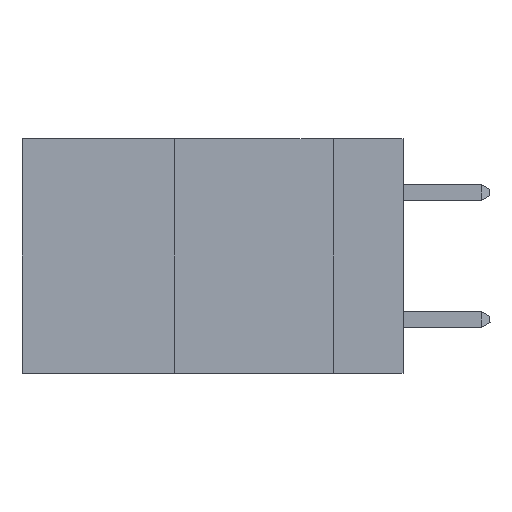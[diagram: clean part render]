
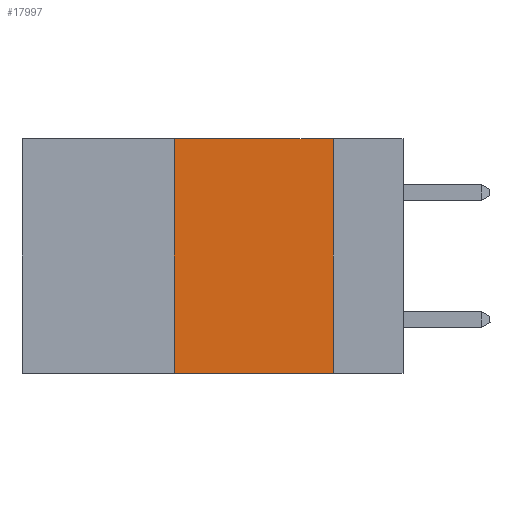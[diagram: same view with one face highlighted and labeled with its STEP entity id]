
A CAD part, left-side view. The second image highlights one B-rep face of the part: STEP entity #17997.
In plain terms, the highlighted planar face has unit normal (-1, 0, 0).
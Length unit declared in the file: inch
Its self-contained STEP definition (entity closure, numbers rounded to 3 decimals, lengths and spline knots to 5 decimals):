
#1113 = DIRECTION ( 'NONE',  ( 0., -1., 0. ) ) ;
#1293 = ORIENTED_EDGE ( 'NONE', *, *, #20661, .T. ) ;
#2357 = LINE ( 'NONE', #15068, #20232 ) ;
#3749 = VECTOR ( 'NONE', #1113, 39.37008 ) ;
#4607 = ORIENTED_EDGE ( 'NONE', *, *, #16120, .F. ) ;
#5428 = CARTESIAN_POINT ( 'NONE',  ( 0., 0.6, -0.37 ) ) ;
#6426 = FACE_OUTER_BOUND ( 'NONE', #14018, .T. ) ;
#7852 = VERTEX_POINT ( 'NONE', #18581 ) ;
#10049 = VERTEX_POINT ( 'NONE', #14645 ) ;
#10486 = DIRECTION ( 'NONE',  ( 0., 0., -1. ) ) ;
#11474 = EDGE_CURVE ( 'NONE', #7852, #10049, #17494, .T. ) ;
#11612 = VERTEX_POINT ( 'NONE', #17171 ) ;
#11817 = DIRECTION ( 'NONE',  ( 0., 0., 1. ) ) ;
#12527 = VECTOR ( 'NONE', #19067, 39.37008 ) ;
#14018 = EDGE_LOOP ( 'NONE', ( #16974, #18585, #4607, #1293 ) ) ;
#14645 = CARTESIAN_POINT ( 'NONE',  ( 0., 0.11, 0. ) ) ;
#15068 = CARTESIAN_POINT ( 'NONE',  ( 0., 0.11, 0. ) ) ;
#15114 = LINE ( 'NONE', #15204, #19676 ) ;
#15204 = CARTESIAN_POINT ( 'NONE',  ( 0., 0.36, 0. ) ) ;
#15254 = EDGE_CURVE ( 'NONE', #10049, #11612, #2357, .T. ) ;
#16120 = EDGE_CURVE ( 'NONE', #21643, #7852, #15114, .T. ) ;
#16174 = AXIS2_PLACEMENT_3D ( 'NONE', #17216, #20624, #10486 ) ;
#16974 = ORIENTED_EDGE ( 'NONE', *, *, #15254, .F. ) ;
#17171 = CARTESIAN_POINT ( 'NONE',  ( 0., 0.11, -0.37 ) ) ;
#17216 = CARTESIAN_POINT ( 'NONE',  ( 0., 0.6, 0. ) ) ;
#17494 = LINE ( 'NONE', #21923, #3749 ) ;
#17997 = ADVANCED_FACE ( 'NONE', ( #6426 ), #22258, .F. ) ;
#18581 = CARTESIAN_POINT ( 'NONE',  ( 0., 0.36, 0. ) ) ;
#18585 = ORIENTED_EDGE ( 'NONE', *, *, #11474, .F. ) ;
#19067 = DIRECTION ( 'NONE',  ( 0., -1., 0. ) ) ;
#19676 = VECTOR ( 'NONE', #11817, 39.37008 ) ;
#19684 = CARTESIAN_POINT ( 'NONE',  ( 0., 0.36, -0.37 ) ) ;
#19807 = DIRECTION ( 'NONE',  ( 0., 0., -1. ) ) ;
#20232 = VECTOR ( 'NONE', #19807, 39.37008 ) ;
#20624 = DIRECTION ( 'NONE',  ( 1., 0., 0. ) ) ;
#20661 = EDGE_CURVE ( 'NONE', #21643, #11612, #21523, .T. ) ;
#21523 = LINE ( 'NONE', #5428, #12527 ) ;
#21643 = VERTEX_POINT ( 'NONE', #19684 ) ;
#21923 = CARTESIAN_POINT ( 'NONE',  ( 0., 0.6, 0. ) ) ;
#22258 = PLANE ( 'NONE',  #16174 ) ;
